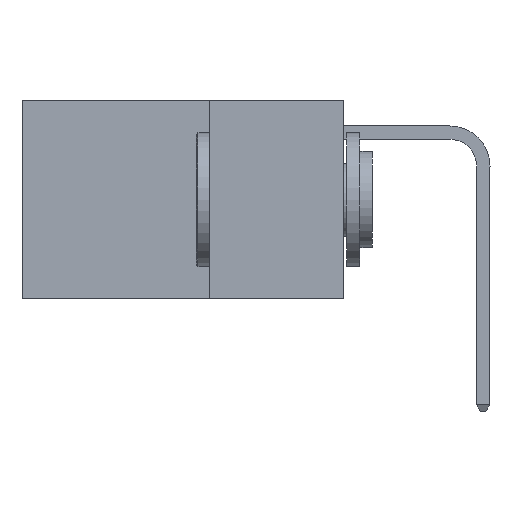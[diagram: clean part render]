
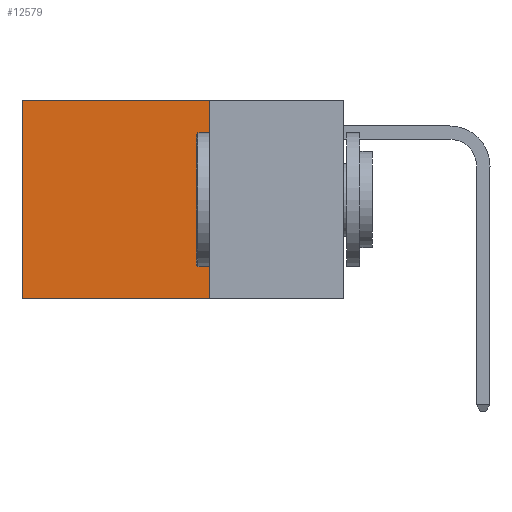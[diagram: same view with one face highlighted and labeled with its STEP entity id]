
A CAD part, left-side view. The second image highlights one B-rep face of the part: STEP entity #12579.
In plain terms, the highlighted planar face has unit normal (-1, 0, 0).
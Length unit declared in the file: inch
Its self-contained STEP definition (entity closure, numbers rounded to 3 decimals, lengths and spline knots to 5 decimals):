
#300 = VECTOR ( 'NONE', #6560, 39.37008 ) ;
#503 = EDGE_CURVE ( 'NONE', #2291, #10524, #13450, .T. ) ;
#1089 = AXIS2_PLACEMENT_3D ( 'NONE', #13627, #14728, #7936 ) ;
#1372 = CARTESIAN_POINT ( 'NONE',  ( 0.2625, 0.6, -0.37 ) ) ;
#1832 = VECTOR ( 'NONE', #6314, 39.37008 ) ;
#2284 = CARTESIAN_POINT ( 'NONE',  ( 0.2625, 0.25, -0.37 ) ) ;
#2291 = VERTEX_POINT ( 'NONE', #7924 ) ;
#2503 = EDGE_CURVE ( 'NONE', #13840, #12187, #9306, .T. ) ;
#3495 = EDGE_CURVE ( 'NONE', #2291, #13840, #4975, .T. ) ;
#3707 = FACE_OUTER_BOUND ( 'NONE', #8162, .T. ) ;
#4253 = DIRECTION ( 'NONE',  ( 0., 0., -1. ) ) ;
#4306 = VECTOR ( 'NONE', #7579, 39.37008 ) ;
#4803 = VECTOR ( 'NONE', #4253, 39.37008 ) ;
#4975 = LINE ( 'NONE', #6371, #1832 ) ;
#4983 = CARTESIAN_POINT ( 'NONE',  ( 0.2625, 0.6, 0. ) ) ;
#6314 = DIRECTION ( 'NONE',  ( 0., 0., -1. ) ) ;
#6371 = CARTESIAN_POINT ( 'NONE',  ( 0.2625, 0.25, 0. ) ) ;
#6526 = ORIENTED_EDGE ( 'NONE', *, *, #3495, .F. ) ;
#6560 = DIRECTION ( 'NONE',  ( 0., 1., 0. ) ) ;
#6615 = CARTESIAN_POINT ( 'NONE',  ( 0.2625, 0.25, -0.37 ) ) ;
#7525 = CARTESIAN_POINT ( 'NONE',  ( 0.2625, 0.25, 0. ) ) ;
#7579 = DIRECTION ( 'NONE',  ( 0., 1., 0. ) ) ;
#7727 = ORIENTED_EDGE ( 'NONE', *, *, #503, .T. ) ;
#7924 = CARTESIAN_POINT ( 'NONE',  ( 0.2625, 0.25, 0. ) ) ;
#7936 = DIRECTION ( 'NONE',  ( 0., 0., -1. ) ) ;
#8162 = EDGE_LOOP ( 'NONE', ( #12035, #11380, #6526, #7727 ) ) ;
#8859 = CARTESIAN_POINT ( 'NONE',  ( 0.2625, 0.6, 0. ) ) ;
#9306 = LINE ( 'NONE', #6615, #300 ) ;
#10524 = VERTEX_POINT ( 'NONE', #4983 ) ;
#11380 = ORIENTED_EDGE ( 'NONE', *, *, #2503, .F. ) ;
#12035 = ORIENTED_EDGE ( 'NONE', *, *, #12450, .T. ) ;
#12187 = VERTEX_POINT ( 'NONE', #1372 ) ;
#12450 = EDGE_CURVE ( 'NONE', #10524, #12187, #13926, .T. ) ;
#12501 = PLANE ( 'NONE',  #1089 ) ;
#12579 = ADVANCED_FACE ( 'NONE', ( #3707 ), #12501, .F. ) ;
#13450 = LINE ( 'NONE', #7525, #4306 ) ;
#13627 = CARTESIAN_POINT ( 'NONE',  ( 0.2625, 0.25, 0. ) ) ;
#13840 = VERTEX_POINT ( 'NONE', #2284 ) ;
#13926 = LINE ( 'NONE', #8859, #4803 ) ;
#14728 = DIRECTION ( 'NONE',  ( 1., 0., 0. ) ) ;
